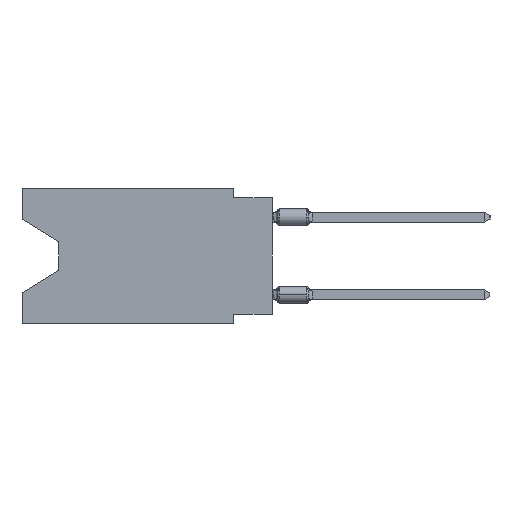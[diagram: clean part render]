
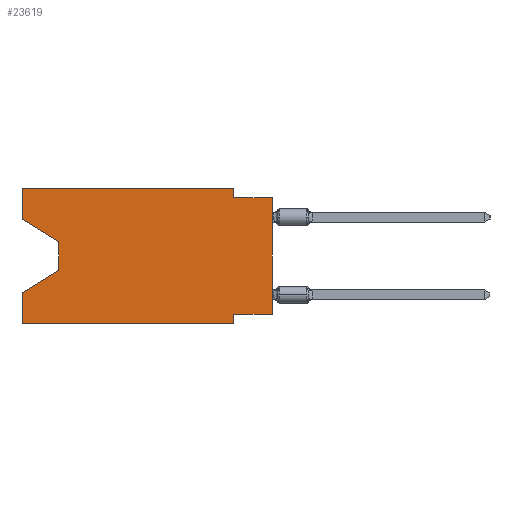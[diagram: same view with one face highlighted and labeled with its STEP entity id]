
A CAD part, left-side view. The second image highlights one B-rep face of the part: STEP entity #23619.
In plain terms, the highlighted planar face has unit normal (-1, 0, 0).
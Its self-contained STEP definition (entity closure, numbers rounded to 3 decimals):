
#85 = CARTESIAN_POINT ( 'NONE',  ( 0., 16.383, 0. ) ) ;
#622 = CARTESIAN_POINT ( 'NONE',  ( 0., 16.383, 0. ) ) ;
#815 = DIRECTION ( 'NONE',  ( 0., 0., -1. ) ) ;
#1837 = CARTESIAN_POINT ( 'NONE',  ( 0., 2.54, 0. ) ) ;
#1915 = ORIENTED_EDGE ( 'NONE', *, *, #5330, .F. ) ;
#2317 = LINE ( 'NONE', #17667, #29022 ) ;
#2570 = LINE ( 'NONE', #12641, #7440 ) ;
#2595 = ORIENTED_EDGE ( 'NONE', *, *, #15870, .T. ) ;
#2907 = LINE ( 'NONE', #12987, #5463 ) ;
#3190 = CARTESIAN_POINT ( 'NONE',  ( 0., 0., 0. ) ) ;
#4037 = ORIENTED_EDGE ( 'NONE', *, *, #13469, .F. ) ;
#4176 = VERTEX_POINT ( 'NONE', #28803 ) ;
#4307 = EDGE_CURVE ( 'NONE', #5804, #6012, #29603, .T. ) ;
#5330 = EDGE_CURVE ( 'NONE', #6012, #8486, #2907, .T. ) ;
#5463 = VECTOR ( 'NONE', #10181, 1000. ) ;
#5766 = LINE ( 'NONE', #23434, #8068 ) ;
#5804 = VERTEX_POINT ( 'NONE', #14178 ) ;
#5813 = CARTESIAN_POINT ( 'NONE',  ( 0., 0., -0.635 ) ) ;
#5822 = CARTESIAN_POINT ( 'NONE',  ( 0., 0., -8.255 ) ) ;
#5911 = EDGE_CURVE ( 'NONE', #29294, #28453, #6905, .T. ) ;
#6012 = VERTEX_POINT ( 'NONE', #28023 ) ;
#6905 = LINE ( 'NONE', #14526, #20278 ) ;
#7046 = EDGE_CURVE ( 'NONE', #18325, #14181, #7814, .T. ) ;
#7411 = DIRECTION ( 'NONE',  ( 0., 0.855, -0.519 ) ) ;
#7440 = VECTOR ( 'NONE', #31371, 1000. ) ;
#7797 = LINE ( 'NONE', #12604, #19864 ) ;
#7814 = LINE ( 'NONE', #20203, #14960 ) ;
#8068 = VECTOR ( 'NONE', #815, 1000. ) ;
#8486 = VERTEX_POINT ( 'NONE', #1837 ) ;
#8559 = DIRECTION ( 'NONE',  ( 0., 1., 0. ) ) ;
#8816 = ORIENTED_EDGE ( 'NONE', *, *, #7046, .F. ) ;
#10031 = VECTOR ( 'NONE', #10288, 1000. ) ;
#10181 = DIRECTION ( 'NONE',  ( 0., -1., 0. ) ) ;
#10288 = DIRECTION ( 'NONE',  ( 0., -1., 0. ) ) ;
#11638 = CARTESIAN_POINT ( 'NONE',  ( 0., 16.383, 0. ) ) ;
#12104 = ORIENTED_EDGE ( 'NONE', *, *, #4307, .F. ) ;
#12400 = DIRECTION ( 'NONE',  ( 0., 0., -1. ) ) ;
#12498 = DIRECTION ( 'NONE',  ( 0., 0., -1. ) ) ;
#12604 = CARTESIAN_POINT ( 'NONE',  ( 0., 13.97, -3.505 ) ) ;
#12622 = DIRECTION ( 'NONE',  ( 0., -1., 0. ) ) ;
#12641 = CARTESIAN_POINT ( 'NONE',  ( 0., 16.383, -2.038 ) ) ;
#12987 = CARTESIAN_POINT ( 'NONE',  ( 0., 16.383, 0. ) ) ;
#13469 = EDGE_CURVE ( 'NONE', #8486, #18325, #5766, .T. ) ;
#14178 = CARTESIAN_POINT ( 'NONE',  ( 0., 16.383, -2.038 ) ) ;
#14181 = VERTEX_POINT ( 'NONE', #5813 ) ;
#14459 = DIRECTION ( 'NONE',  ( 0., 0., 1. ) ) ;
#14526 = CARTESIAN_POINT ( 'NONE',  ( 0., 13.97, -5.385 ) ) ;
#14960 = VECTOR ( 'NONE', #12622, 1000. ) ;
#15142 = PLANE ( 'NONE',  #22877 ) ;
#15405 = CARTESIAN_POINT ( 'NONE',  ( 0., 16.383, -8.89 ) ) ;
#15809 = CARTESIAN_POINT ( 'NONE',  ( 0., 2.54, -0.635 ) ) ;
#15839 = DIRECTION ( 'NONE',  ( 0., 0., 1. ) ) ;
#15870 = EDGE_CURVE ( 'NONE', #18508, #14181, #18210, .T. ) ;
#16081 = DIRECTION ( 'NONE',  ( 0., 0., 1. ) ) ;
#16169 = LINE ( 'NONE', #29005, #18060 ) ;
#17029 = EDGE_CURVE ( 'NONE', #5804, #4176, #2570, .T. ) ;
#17667 = CARTESIAN_POINT ( 'NONE',  ( 0., 2.54, -8.89 ) ) ;
#17763 = DIRECTION ( 'NONE',  ( 1., 0., 0. ) ) ;
#18060 = VECTOR ( 'NONE', #8559, 1000. ) ;
#18195 = ORIENTED_EDGE ( 'NONE', *, *, #5911, .T. ) ;
#18210 = LINE ( 'NONE', #3190, #21075 ) ;
#18325 = VERTEX_POINT ( 'NONE', #15809 ) ;
#18508 = VERTEX_POINT ( 'NONE', #5822 ) ;
#19335 = ORIENTED_EDGE ( 'NONE', *, *, #21549, .F. ) ;
#19864 = VECTOR ( 'NONE', #30237, 1000. ) ;
#19882 = ORIENTED_EDGE ( 'NONE', *, *, #30670, .F. ) ;
#20203 = CARTESIAN_POINT ( 'NONE',  ( 0., 0., -0.635 ) ) ;
#20278 = VECTOR ( 'NONE', #7411, 1000. ) ;
#20498 = CARTESIAN_POINT ( 'NONE',  ( 0., 16.383, -8.89 ) ) ;
#20843 = ORIENTED_EDGE ( 'NONE', *, *, #31793, .T. ) ;
#21075 = VECTOR ( 'NONE', #16081, 1000. ) ;
#21549 = EDGE_CURVE ( 'NONE', #18508, #26725, #16169, .T. ) ;
#21862 = CARTESIAN_POINT ( 'NONE',  ( 0., 2.54, -8.89 ) ) ;
#22631 = ORIENTED_EDGE ( 'NONE', *, *, #17029, .T. ) ;
#22658 = LINE ( 'NONE', #15405, #10031 ) ;
#22877 = AXIS2_PLACEMENT_3D ( 'NONE', #85, #17763, #12498 ) ;
#23434 = CARTESIAN_POINT ( 'NONE',  ( 0., 2.54, 0. ) ) ;
#23619 = ADVANCED_FACE ( 'NONE', ( #25336 ), #15142, .F. ) ;
#24068 = EDGE_CURVE ( 'NONE', #4176, #29294, #7797, .T. ) ;
#24569 = EDGE_LOOP ( 'NONE', ( #22631, #28473, #18195, #19882, #20843, #31435, #19335, #2595, #8816, #4037, #1915, #12104 ) ) ;
#25336 = FACE_OUTER_BOUND ( 'NONE', #24569, .T. ) ;
#25373 = VECTOR ( 'NONE', #15839, 1000. ) ;
#25675 = CARTESIAN_POINT ( 'NONE',  ( 0., 2.54, -8.255 ) ) ;
#26229 = VERTEX_POINT ( 'NONE', #21862 ) ;
#26725 = VERTEX_POINT ( 'NONE', #25675 ) ;
#27092 = VECTOR ( 'NONE', #14459, 1000. ) ;
#27720 = CARTESIAN_POINT ( 'NONE',  ( 0., 13.97, -5.385 ) ) ;
#28023 = CARTESIAN_POINT ( 'NONE',  ( 0., 16.383, 0. ) ) ;
#28034 = LINE ( 'NONE', #622, #25373 ) ;
#28453 = VERTEX_POINT ( 'NONE', #31514 ) ;
#28473 = ORIENTED_EDGE ( 'NONE', *, *, #24068, .T. ) ;
#28803 = CARTESIAN_POINT ( 'NONE',  ( 0., 13.97, -3.505 ) ) ;
#29005 = CARTESIAN_POINT ( 'NONE',  ( 0., 0., -8.255 ) ) ;
#29022 = VECTOR ( 'NONE', #12400, 1000. ) ;
#29294 = VERTEX_POINT ( 'NONE', #27720 ) ;
#29603 = LINE ( 'NONE', #11638, #27092 ) ;
#30237 = DIRECTION ( 'NONE',  ( 0., 0., -1. ) ) ;
#30479 = EDGE_CURVE ( 'NONE', #26725, #26229, #2317, .T. ) ;
#30670 = EDGE_CURVE ( 'NONE', #31746, #28453, #28034, .T. ) ;
#31371 = DIRECTION ( 'NONE',  ( 0., -0.855, -0.519 ) ) ;
#31435 = ORIENTED_EDGE ( 'NONE', *, *, #30479, .F. ) ;
#31514 = CARTESIAN_POINT ( 'NONE',  ( 0., 16.383, -6.852 ) ) ;
#31746 = VERTEX_POINT ( 'NONE', #20498 ) ;
#31793 = EDGE_CURVE ( 'NONE', #31746, #26229, #22658, .T. ) ;
